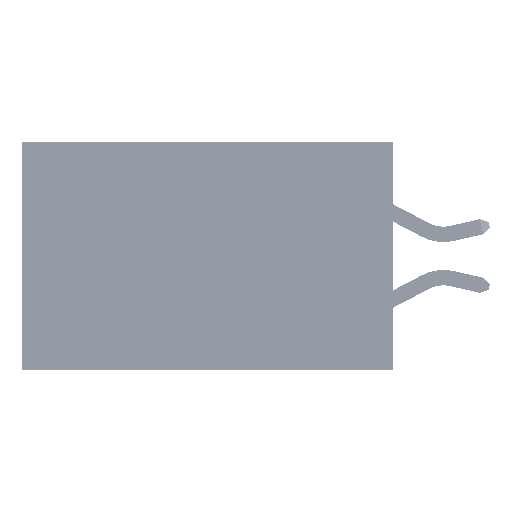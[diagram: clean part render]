
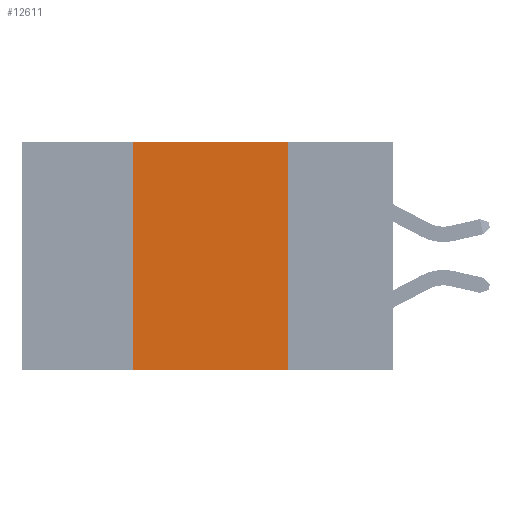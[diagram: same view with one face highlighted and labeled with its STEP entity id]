
A CAD part, left-side view. The second image highlights one B-rep face of the part: STEP entity #12611.
In plain terms, the highlighted planar face has unit normal (-1, 0, 0).
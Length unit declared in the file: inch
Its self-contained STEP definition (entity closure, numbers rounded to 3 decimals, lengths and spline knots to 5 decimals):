
#3294 = EDGE_CURVE ( 'NONE', #28274, #40811, #30084, .T. ) ;
#4840 = AXIS2_PLACEMENT_3D ( 'NONE', #12840, #34821, #16335 ) ;
#7026 = ORIENTED_EDGE ( 'NONE', *, *, #3294, .F. ) ;
#7849 = CARTESIAN_POINT ( 'NONE',  ( 0., 0.17, 0. ) ) ;
#8351 = EDGE_CURVE ( 'NONE', #18364, #28274, #9321, .T. ) ;
#8535 = EDGE_CURVE ( 'NONE', #40811, #21470, #11302, .T. ) ;
#9321 = LINE ( 'NONE', #47798, #34953 ) ;
#9707 = CARTESIAN_POINT ( 'NONE',  ( 0., 0.6, -0.37 ) ) ;
#10672 = EDGE_CURVE ( 'NONE', #18364, #21470, #41140, .T. ) ;
#11048 = CARTESIAN_POINT ( 'NONE',  ( 0., 0.17, 0. ) ) ;
#11302 = LINE ( 'NONE', #11048, #31000 ) ;
#12611 = ADVANCED_FACE ( 'NONE', ( #19585 ), #24315, .F. ) ;
#12840 = CARTESIAN_POINT ( 'NONE',  ( 0., 0.6, 0. ) ) ;
#14441 = EDGE_LOOP ( 'NONE', ( #26961, #7026, #23676, #45389 ) ) ;
#16335 = DIRECTION ( 'NONE',  ( 0., 0., -1. ) ) ;
#18364 = VERTEX_POINT ( 'NONE', #25789 ) ;
#19585 = FACE_OUTER_BOUND ( 'NONE', #14441, .T. ) ;
#21470 = VERTEX_POINT ( 'NONE', #38219 ) ;
#23676 = ORIENTED_EDGE ( 'NONE', *, *, #8351, .F. ) ;
#24315 = PLANE ( 'NONE',  #4840 ) ;
#25789 = CARTESIAN_POINT ( 'NONE',  ( 0., 0.42, -0.37 ) ) ;
#26868 = VECTOR ( 'NONE', #37146, 39.37008 ) ;
#26961 = ORIENTED_EDGE ( 'NONE', *, *, #8535, .F. ) ;
#28274 = VERTEX_POINT ( 'NONE', #45401 ) ;
#30084 = LINE ( 'NONE', #44337, #31456 ) ;
#31000 = VECTOR ( 'NONE', #44519, 39.37008 ) ;
#31456 = VECTOR ( 'NONE', #45321, 39.37008 ) ;
#34821 = DIRECTION ( 'NONE',  ( 1., 0., 0. ) ) ;
#34953 = VECTOR ( 'NONE', #43781, 39.37008 ) ;
#37146 = DIRECTION ( 'NONE',  ( 0., -1., 0. ) ) ;
#38219 = CARTESIAN_POINT ( 'NONE',  ( 0., 0.17, -0.37 ) ) ;
#40811 = VERTEX_POINT ( 'NONE', #7849 ) ;
#41140 = LINE ( 'NONE', #9707, #26868 ) ;
#43781 = DIRECTION ( 'NONE',  ( 0., 0., 1. ) ) ;
#44337 = CARTESIAN_POINT ( 'NONE',  ( 0., 0.6, 0. ) ) ;
#44519 = DIRECTION ( 'NONE',  ( 0., 0., -1. ) ) ;
#45321 = DIRECTION ( 'NONE',  ( 0., -1., 0. ) ) ;
#45389 = ORIENTED_EDGE ( 'NONE', *, *, #10672, .T. ) ;
#45401 = CARTESIAN_POINT ( 'NONE',  ( 0., 0.42, 0. ) ) ;
#47798 = CARTESIAN_POINT ( 'NONE',  ( 0., 0.42, 0. ) ) ;
